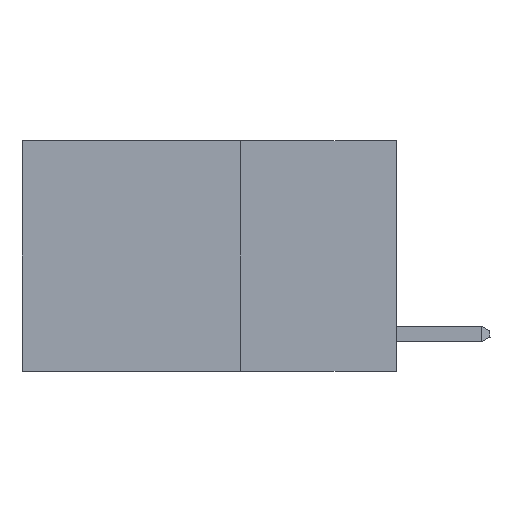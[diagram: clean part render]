
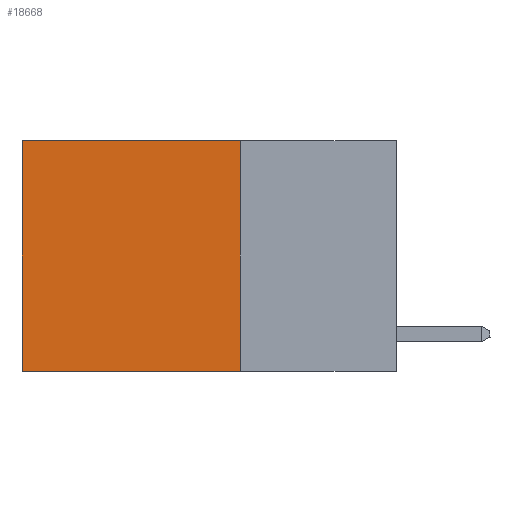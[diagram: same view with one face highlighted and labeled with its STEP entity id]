
A CAD part, left-side view. The second image highlights one B-rep face of the part: STEP entity #18668.
In plain terms, the highlighted planar face has unit normal (-1, 0, 0).
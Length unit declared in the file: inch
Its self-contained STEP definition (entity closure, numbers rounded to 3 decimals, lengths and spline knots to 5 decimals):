
#1037 = LINE ( 'NONE', #23633, #19818 ) ;
#1378 = VERTEX_POINT ( 'NONE', #21627 ) ;
#4312 = ORIENTED_EDGE ( 'NONE', *, *, #15506, .T. ) ;
#5712 = CARTESIAN_POINT ( 'NONE',  ( 0.2625, 0.25, -0.37 ) ) ;
#6979 = EDGE_CURVE ( 'NONE', #1378, #11281, #12304, .T. ) ;
#7093 = CARTESIAN_POINT ( 'NONE',  ( 0.2625, 0.25, 0. ) ) ;
#7256 = CARTESIAN_POINT ( 'NONE',  ( 0.2625, 0.6, 0. ) ) ;
#7317 = VECTOR ( 'NONE', #11378, 39.37008 ) ;
#8019 = LINE ( 'NONE', #23465, #12971 ) ;
#9727 = LINE ( 'NONE', #7093, #19086 ) ;
#10263 = VERTEX_POINT ( 'NONE', #22430 ) ;
#10572 = DIRECTION ( 'NONE',  ( 0., 1., 0. ) ) ;
#11126 = DIRECTION ( 'NONE',  ( 0., 0., -1. ) ) ;
#11281 = VERTEX_POINT ( 'NONE', #21502 ) ;
#11378 = DIRECTION ( 'NONE',  ( 0., 1., 0. ) ) ;
#11645 = AXIS2_PLACEMENT_3D ( 'NONE', #16686, #22365, #11126 ) ;
#12304 = LINE ( 'NONE', #5712, #7317 ) ;
#12809 = VERTEX_POINT ( 'NONE', #7256 ) ;
#12971 = VECTOR ( 'NONE', #14076, 39.37008 ) ;
#14076 = DIRECTION ( 'NONE',  ( 0., 0., -1. ) ) ;
#15506 = EDGE_CURVE ( 'NONE', #10263, #12809, #1037, .T. ) ;
#16686 = CARTESIAN_POINT ( 'NONE',  ( 0.2625, 0.25, 0. ) ) ;
#16914 = ORIENTED_EDGE ( 'NONE', *, *, #20878, .F. ) ;
#18668 = ADVANCED_FACE ( 'NONE', ( #24233 ), #20380, .F. ) ;
#19086 = VECTOR ( 'NONE', #22092, 39.37008 ) ;
#19818 = VECTOR ( 'NONE', #10572, 39.37008 ) ;
#20038 = EDGE_CURVE ( 'NONE', #12809, #11281, #8019, .T. ) ;
#20380 = PLANE ( 'NONE',  #11645 ) ;
#20452 = ORIENTED_EDGE ( 'NONE', *, *, #20038, .T. ) ;
#20878 = EDGE_CURVE ( 'NONE', #10263, #1378, #9727, .T. ) ;
#21303 = EDGE_LOOP ( 'NONE', ( #20452, #22921, #16914, #4312 ) ) ;
#21502 = CARTESIAN_POINT ( 'NONE',  ( 0.2625, 0.6, -0.37 ) ) ;
#21627 = CARTESIAN_POINT ( 'NONE',  ( 0.2625, 0.25, -0.37 ) ) ;
#22092 = DIRECTION ( 'NONE',  ( 0., 0., -1. ) ) ;
#22365 = DIRECTION ( 'NONE',  ( 1., 0., 0. ) ) ;
#22430 = CARTESIAN_POINT ( 'NONE',  ( 0.2625, 0.25, 0. ) ) ;
#22921 = ORIENTED_EDGE ( 'NONE', *, *, #6979, .F. ) ;
#23465 = CARTESIAN_POINT ( 'NONE',  ( 0.2625, 0.6, 0. ) ) ;
#23633 = CARTESIAN_POINT ( 'NONE',  ( 0.2625, 0.25, 0. ) ) ;
#24233 = FACE_OUTER_BOUND ( 'NONE', #21303, .T. ) ;
